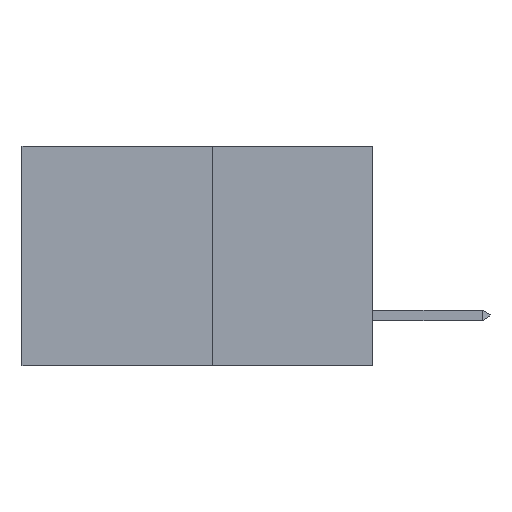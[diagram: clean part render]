
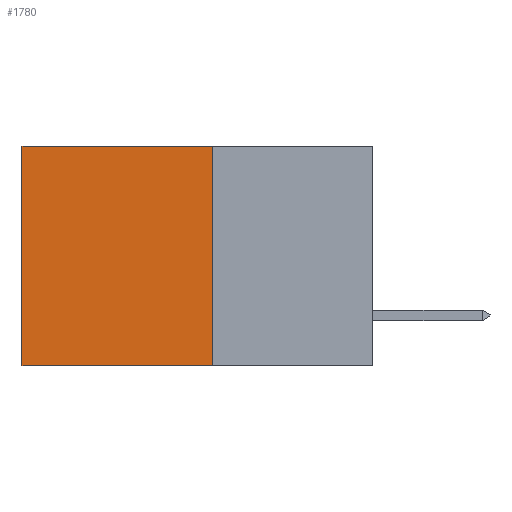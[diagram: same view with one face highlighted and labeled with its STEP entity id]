
A CAD part, left-side view. The second image highlights one B-rep face of the part: STEP entity #1780.
In plain terms, the highlighted planar face has unit normal (-1, 0, 0).
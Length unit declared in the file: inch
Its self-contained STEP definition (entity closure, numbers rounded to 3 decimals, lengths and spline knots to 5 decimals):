
#206 = DIRECTION ( 'NONE',  ( 0., 0., -1. ) ) ;
#233 = VECTOR ( 'NONE', #3989, 39.37008 ) ;
#398 = EDGE_CURVE ( 'NONE', #8516, #9172, #6743, .T. ) ;
#536 = CARTESIAN_POINT ( 'NONE',  ( 0.277, 0.27, 0. ) ) ;
#575 = LINE ( 'NONE', #6259, #233 ) ;
#1159 = ORIENTED_EDGE ( 'NONE', *, *, #5037, .T. ) ;
#1242 = CARTESIAN_POINT ( 'NONE',  ( 0.277, 0.59, -0.37 ) ) ;
#1586 = CARTESIAN_POINT ( 'NONE',  ( 0.277, 0.27, -0.37 ) ) ;
#1780 = ADVANCED_FACE ( 'NONE', ( #8136 ), #6045, .F. ) ;
#2241 = CARTESIAN_POINT ( 'NONE',  ( 0.277, 0.27, -0.37 ) ) ;
#2600 = AXIS2_PLACEMENT_3D ( 'NONE', #1586, #8797, #3258 ) ;
#2698 = EDGE_CURVE ( 'NONE', #9172, #5710, #4574, .T. ) ;
#3258 = DIRECTION ( 'NONE',  ( 0., 0., -1. ) ) ;
#3273 = EDGE_CURVE ( 'NONE', #5775, #5710, #7028, .T. ) ;
#3859 = ORIENTED_EDGE ( 'NONE', *, *, #3273, .T. ) ;
#3975 = ORIENTED_EDGE ( 'NONE', *, *, #398, .F. ) ;
#3989 = DIRECTION ( 'NONE',  ( 0., 1., 0. ) ) ;
#3991 = DIRECTION ( 'NONE',  ( 0., 1., 0. ) ) ;
#4238 = ORIENTED_EDGE ( 'NONE', *, *, #2698, .F. ) ;
#4574 = LINE ( 'NONE', #2241, #8462 ) ;
#4767 = CARTESIAN_POINT ( 'NONE',  ( 0.277, 0.59, 0. ) ) ;
#4922 = VECTOR ( 'NONE', #9476, 39.37008 ) ;
#4960 = CARTESIAN_POINT ( 'NONE',  ( 0.277, 0.59, -0.37 ) ) ;
#5037 = EDGE_CURVE ( 'NONE', #8516, #5775, #575, .T. ) ;
#5596 = CARTESIAN_POINT ( 'NONE',  ( 0.277, 0.27, -0.37 ) ) ;
#5710 = VERTEX_POINT ( 'NONE', #4960 ) ;
#5775 = VERTEX_POINT ( 'NONE', #4767 ) ;
#6045 = PLANE ( 'NONE',  #2600 ) ;
#6259 = CARTESIAN_POINT ( 'NONE',  ( 0.277, 0.27, 0. ) ) ;
#6743 = LINE ( 'NONE', #5596, #4922 ) ;
#7028 = LINE ( 'NONE', #1242, #8793 ) ;
#7115 = CARTESIAN_POINT ( 'NONE',  ( 0.277, 0.27, -0.37 ) ) ;
#7586 = EDGE_LOOP ( 'NONE', ( #3859, #4238, #3975, #1159 ) ) ;
#8136 = FACE_OUTER_BOUND ( 'NONE', #7586, .T. ) ;
#8462 = VECTOR ( 'NONE', #3991, 39.37008 ) ;
#8516 = VERTEX_POINT ( 'NONE', #536 ) ;
#8793 = VECTOR ( 'NONE', #206, 39.37008 ) ;
#8797 = DIRECTION ( 'NONE',  ( 1., 0., 0. ) ) ;
#9172 = VERTEX_POINT ( 'NONE', #7115 ) ;
#9476 = DIRECTION ( 'NONE',  ( 0., 0., -1. ) ) ;
